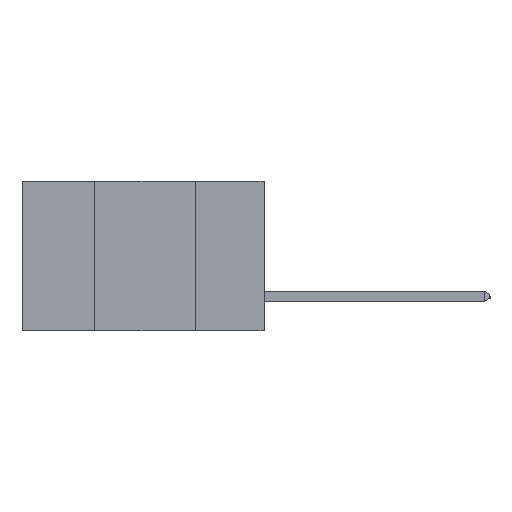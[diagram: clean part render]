
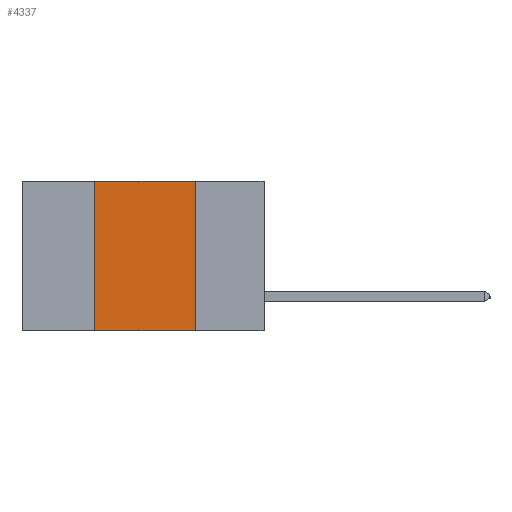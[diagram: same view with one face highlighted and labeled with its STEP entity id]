
A CAD part, left-side view. The second image highlights one B-rep face of the part: STEP entity #4337.
In plain terms, the highlighted planar face has unit normal (-1, 0, 0).
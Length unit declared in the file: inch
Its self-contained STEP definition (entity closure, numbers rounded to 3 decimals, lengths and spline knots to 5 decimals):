
#331 = PLANE ( 'NONE',  #2228 ) ;
#490 = DIRECTION ( 'NONE',  ( 0., 0., 1. ) ) ;
#516 = LINE ( 'NONE', #7181, #3464 ) ;
#1118 = ORIENTED_EDGE ( 'NONE', *, *, #2896, .F. ) ;
#1285 = LINE ( 'NONE', #9182, #10478 ) ;
#1770 = CARTESIAN_POINT ( 'NONE',  ( 0., 0.6, 0. ) ) ;
#1999 = VECTOR ( 'NONE', #6708, 39.37008 ) ;
#2228 = AXIS2_PLACEMENT_3D ( 'NONE', #1770, #11214, #3048 ) ;
#2640 = ORIENTED_EDGE ( 'NONE', *, *, #4991, .T. ) ;
#2810 = LINE ( 'NONE', #14728, #1999 ) ;
#2837 = CARTESIAN_POINT ( 'NONE',  ( 0., 0.42, -0.37 ) ) ;
#2896 = EDGE_CURVE ( 'NONE', #4423, #9780, #8225, .T. ) ;
#3048 = DIRECTION ( 'NONE',  ( 0., 0., -1. ) ) ;
#3360 = CARTESIAN_POINT ( 'NONE',  ( 0., 0.42, 0. ) ) ;
#3366 = CARTESIAN_POINT ( 'NONE',  ( 0., 0.17, -0.37 ) ) ;
#3464 = VECTOR ( 'NONE', #10654, 39.37008 ) ;
#4337 = ADVANCED_FACE ( 'NONE', ( #11779 ), #331, .F. ) ;
#4423 = VERTEX_POINT ( 'NONE', #2837 ) ;
#4456 = VERTEX_POINT ( 'NONE', #3366 ) ;
#4991 = EDGE_CURVE ( 'NONE', #4423, #4456, #1285, .T. ) ;
#5048 = DIRECTION ( 'NONE',  ( 0., -1., 0. ) ) ;
#5858 = ORIENTED_EDGE ( 'NONE', *, *, #12506, .F. ) ;
#6708 = DIRECTION ( 'NONE',  ( 0., -1., 0. ) ) ;
#6864 = ORIENTED_EDGE ( 'NONE', *, *, #13855, .F. ) ;
#7181 = CARTESIAN_POINT ( 'NONE',  ( 0., 0.17, 0. ) ) ;
#8225 = LINE ( 'NONE', #3360, #10936 ) ;
#9182 = CARTESIAN_POINT ( 'NONE',  ( 0., 0.6, -0.37 ) ) ;
#9780 = VERTEX_POINT ( 'NONE', #12931 ) ;
#10356 = VERTEX_POINT ( 'NONE', #12797 ) ;
#10478 = VECTOR ( 'NONE', #5048, 39.37008 ) ;
#10654 = DIRECTION ( 'NONE',  ( 0., 0., -1. ) ) ;
#10936 = VECTOR ( 'NONE', #490, 39.37008 ) ;
#11214 = DIRECTION ( 'NONE',  ( 1., 0., 0. ) ) ;
#11779 = FACE_OUTER_BOUND ( 'NONE', #13766, .T. ) ;
#12506 = EDGE_CURVE ( 'NONE', #10356, #4456, #516, .T. ) ;
#12797 = CARTESIAN_POINT ( 'NONE',  ( 0., 0.17, 0. ) ) ;
#12931 = CARTESIAN_POINT ( 'NONE',  ( 0., 0.42, 0. ) ) ;
#13766 = EDGE_LOOP ( 'NONE', ( #5858, #6864, #1118, #2640 ) ) ;
#13855 = EDGE_CURVE ( 'NONE', #9780, #10356, #2810, .T. ) ;
#14728 = CARTESIAN_POINT ( 'NONE',  ( 0., 0.6, 0. ) ) ;
